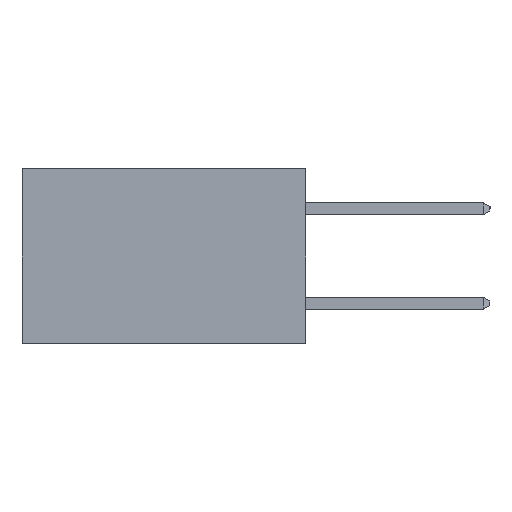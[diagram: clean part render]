
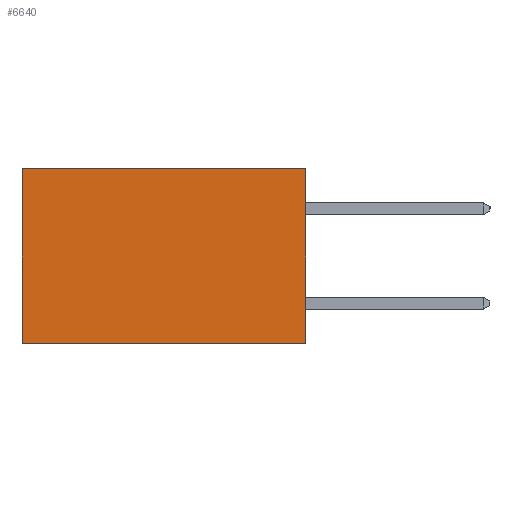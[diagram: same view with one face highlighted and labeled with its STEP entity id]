
A CAD part, left-side view. The second image highlights one B-rep face of the part: STEP entity #6640.
In plain terms, the highlighted planar face has unit normal (-1, 0, 0).
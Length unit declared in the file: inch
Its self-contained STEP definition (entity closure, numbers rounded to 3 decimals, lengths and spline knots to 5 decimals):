
#158 = ORIENTED_EDGE ( 'NONE', *, *, #11435, .T. ) ;
#206 = CARTESIAN_POINT ( 'NONE',  ( 0.2615, 0., -0.37 ) ) ;
#414 = CARTESIAN_POINT ( 'NONE',  ( 0.2615, 0., -0.37 ) ) ;
#784 = CARTESIAN_POINT ( 'NONE',  ( 0.2615, 0.6, 0. ) ) ;
#790 = LINE ( 'NONE', #3919, #1762 ) ;
#809 = CARTESIAN_POINT ( 'NONE',  ( 0.2615, 0., -0.37 ) ) ;
#1422 = EDGE_CURVE ( 'NONE', #1775, #2579, #2943, .T. ) ;
#1762 = VECTOR ( 'NONE', #5786, 39.37008 ) ;
#1775 = VERTEX_POINT ( 'NONE', #10252 ) ;
#1849 = CARTESIAN_POINT ( 'NONE',  ( 0.2615, 0.6, -0.37 ) ) ;
#2579 = VERTEX_POINT ( 'NONE', #784 ) ;
#2736 = PLANE ( 'NONE',  #3293 ) ;
#2943 = LINE ( 'NONE', #11108, #6022 ) ;
#3293 = AXIS2_PLACEMENT_3D ( 'NONE', #809, #7244, #6339 ) ;
#3495 = DIRECTION ( 'NONE',  ( 0., 0., -1. ) ) ;
#3919 = CARTESIAN_POINT ( 'NONE',  ( 0.2615, 0., -0.37 ) ) ;
#4068 = ORIENTED_EDGE ( 'NONE', *, *, #5854, .F. ) ;
#4340 = LINE ( 'NONE', #8009, #9735 ) ;
#4439 = VERTEX_POINT ( 'NONE', #1849 ) ;
#4508 = ORIENTED_EDGE ( 'NONE', *, *, #1422, .T. ) ;
#4899 = DIRECTION ( 'NONE',  ( 0., 1., 0. ) ) ;
#5786 = DIRECTION ( 'NONE',  ( 0., 0., -1. ) ) ;
#5854 = EDGE_CURVE ( 'NONE', #1775, #10081, #790, .T. ) ;
#6022 = VECTOR ( 'NONE', #10268, 39.37008 ) ;
#6339 = DIRECTION ( 'NONE',  ( 0., 0., -1. ) ) ;
#6460 = FACE_OUTER_BOUND ( 'NONE', #7685, .T. ) ;
#6640 = ADVANCED_FACE ( 'NONE', ( #6460 ), #2736, .F. ) ;
#7244 = DIRECTION ( 'NONE',  ( 1., 0., 0. ) ) ;
#7616 = VECTOR ( 'NONE', #4899, 39.37008 ) ;
#7685 = EDGE_LOOP ( 'NONE', ( #158, #8492, #4068, #4508 ) ) ;
#8009 = CARTESIAN_POINT ( 'NONE',  ( 0.2615, 0.6, -0.37 ) ) ;
#8492 = ORIENTED_EDGE ( 'NONE', *, *, #10916, .F. ) ;
#9735 = VECTOR ( 'NONE', #3495, 39.37008 ) ;
#10081 = VERTEX_POINT ( 'NONE', #414 ) ;
#10252 = CARTESIAN_POINT ( 'NONE',  ( 0.2615, 0., 0. ) ) ;
#10268 = DIRECTION ( 'NONE',  ( 0., 1., 0. ) ) ;
#10916 = EDGE_CURVE ( 'NONE', #10081, #4439, #11327, .T. ) ;
#11108 = CARTESIAN_POINT ( 'NONE',  ( 0.2615, 0., 0. ) ) ;
#11327 = LINE ( 'NONE', #206, #7616 ) ;
#11435 = EDGE_CURVE ( 'NONE', #2579, #4439, #4340, .T. ) ;
